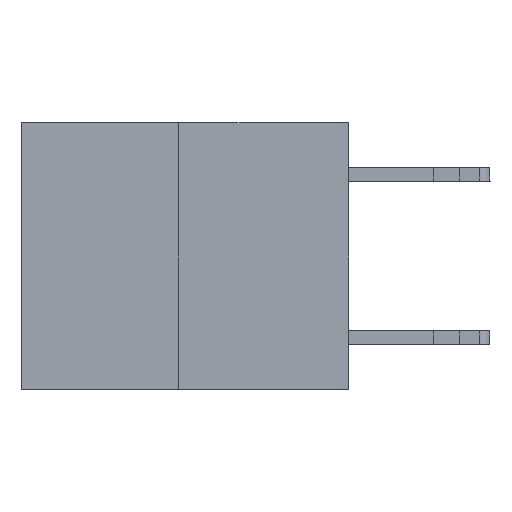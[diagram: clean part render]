
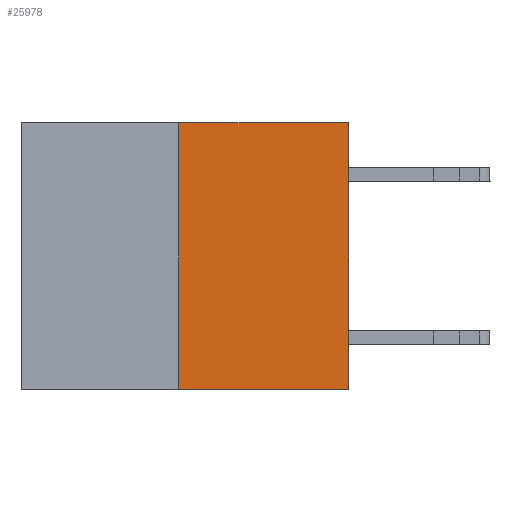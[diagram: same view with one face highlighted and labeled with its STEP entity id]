
A CAD part, left-side view. The second image highlights one B-rep face of the part: STEP entity #25978.
In plain terms, the highlighted planar face has unit normal (-1, 0, 0).
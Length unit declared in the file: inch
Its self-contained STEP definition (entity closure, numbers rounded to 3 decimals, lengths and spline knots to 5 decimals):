
#162 = EDGE_CURVE ( 'NONE', #23133, #7816, #7458, .T. ) ;
#1723 = EDGE_CURVE ( 'NONE', #6893, #14950, #24713, .T. ) ;
#2134 = CARTESIAN_POINT ( 'NONE',  ( 0., 0.312, 0. ) ) ;
#3301 = CARTESIAN_POINT ( 'NONE',  ( 0., 0.312, -0.49 ) ) ;
#3528 = CARTESIAN_POINT ( 'NONE',  ( 0., 0.6, 0. ) ) ;
#3630 = FACE_OUTER_BOUND ( 'NONE', #12186, .T. ) ;
#3860 = VECTOR ( 'NONE', #5363, 39.37008 ) ;
#4039 = AXIS2_PLACEMENT_3D ( 'NONE', #3528, #11786, #21956 ) ;
#4180 = CARTESIAN_POINT ( 'NONE',  ( 0., 0.6, 0. ) ) ;
#5363 = DIRECTION ( 'NONE',  ( 0., 0., 1. ) ) ;
#5972 = CARTESIAN_POINT ( 'NONE',  ( 0., 0., 0. ) ) ;
#6893 = VERTEX_POINT ( 'NONE', #2134 ) ;
#7458 = LINE ( 'NONE', #23926, #23124 ) ;
#7555 = CARTESIAN_POINT ( 'NONE',  ( 0., 0.312, -0.49 ) ) ;
#7816 = VERTEX_POINT ( 'NONE', #9169 ) ;
#8128 = CARTESIAN_POINT ( 'NONE',  ( 0., 0., 0. ) ) ;
#8846 = EDGE_CURVE ( 'NONE', #7816, #14950, #11048, .T. ) ;
#9169 = CARTESIAN_POINT ( 'NONE',  ( 0., 0., -0.49 ) ) ;
#9569 = ORIENTED_EDGE ( 'NONE', *, *, #1723, .F. ) ;
#10070 = VECTOR ( 'NONE', #18709, 39.37008 ) ;
#11048 = LINE ( 'NONE', #5972, #10070 ) ;
#11387 = EDGE_CURVE ( 'NONE', #23133, #6893, #18911, .T. ) ;
#11437 = DIRECTION ( 'NONE',  ( 0., -1., 0. ) ) ;
#11786 = DIRECTION ( 'NONE',  ( 1., 0., 0. ) ) ;
#12186 = EDGE_LOOP ( 'NONE', ( #20192, #25570, #23366, #9569 ) ) ;
#14950 = VERTEX_POINT ( 'NONE', #8128 ) ;
#18709 = DIRECTION ( 'NONE',  ( 0., 0., 1. ) ) ;
#18728 = DIRECTION ( 'NONE',  ( 0., -1., 0. ) ) ;
#18911 = LINE ( 'NONE', #3301, #3860 ) ;
#20192 = ORIENTED_EDGE ( 'NONE', *, *, #11387, .F. ) ;
#20746 = VECTOR ( 'NONE', #18728, 39.37008 ) ;
#21956 = DIRECTION ( 'NONE',  ( 0., 0., -1. ) ) ;
#23124 = VECTOR ( 'NONE', #11437, 39.37008 ) ;
#23133 = VERTEX_POINT ( 'NONE', #7555 ) ;
#23366 = ORIENTED_EDGE ( 'NONE', *, *, #8846, .T. ) ;
#23926 = CARTESIAN_POINT ( 'NONE',  ( 0., 0.6, -0.49 ) ) ;
#24713 = LINE ( 'NONE', #4180, #20746 ) ;
#25570 = ORIENTED_EDGE ( 'NONE', *, *, #162, .T. ) ;
#25978 = ADVANCED_FACE ( 'NONE', ( #3630 ), #26500, .F. ) ;
#26500 = PLANE ( 'NONE',  #4039 ) ;
